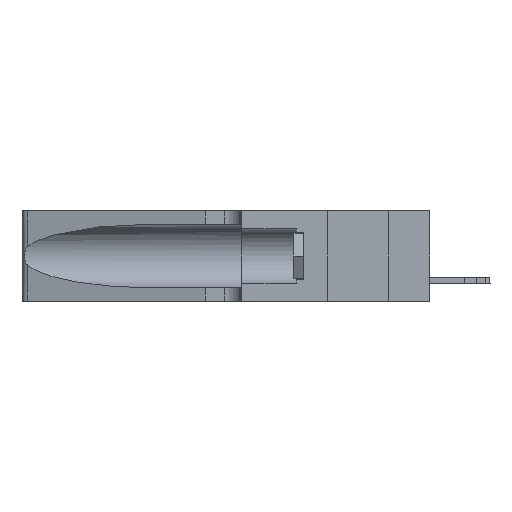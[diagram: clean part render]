
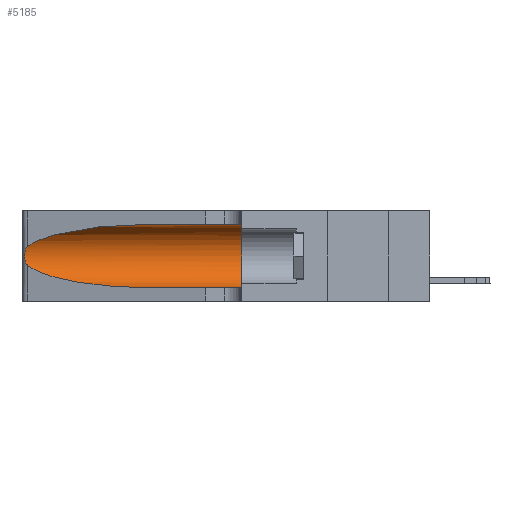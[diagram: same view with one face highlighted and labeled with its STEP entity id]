
A CAD part, left-side view. The second image highlights one B-rep face of the part: STEP entity #5185.
In plain terms, the highlighted cylindrical face has radius 3.308 mm (diameter 6.617 mm), a partial arc.
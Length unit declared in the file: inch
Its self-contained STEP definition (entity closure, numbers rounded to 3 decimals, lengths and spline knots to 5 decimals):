
#22 = CARTESIAN_POINT ( 'NONE',  ( 0.25789, 1.23486, 0.15765 ) ) ;
#763 = DIRECTION ( 'NONE',  ( 0., -1., 0. ) ) ;
#1405 = ORIENTED_EDGE ( 'NONE', *, *, #16992, .T. ) ;
#1784 = CYLINDRICAL_SURFACE ( 'NONE', #16320, 0.13025 ) ;
#2028 = CARTESIAN_POINT ( 'NONE',  ( 0.1305, 0.72297, 0.31525 ) ) ;
#2311 = VECTOR ( 'NONE', #4547, 39.37008 ) ;
#2372 = CARTESIAN_POINT ( 'NONE',  ( 0.25487, 1.22718, 0.22369 ) ) ;
#2548 = EDGE_CURVE ( 'NONE', #8157, #13876, #9603, .T. ) ;
#2886 = CARTESIAN_POINT ( 'NONE',  ( 0.2373, 1.15595, 0.08982 ) ) ;
#3053 = CARTESIAN_POINT ( 'NONE',  ( 0.1305, 0.72297, 0.05475 ) ) ;
#3152 = CARTESIAN_POINT ( 'NONE',  ( 0.18966, 0.96281, 0.05475 ) ) ;
#3193 = EDGE_CURVE ( 'NONE', #5038, #15897, #12109, .T. ) ;
#4183 = EDGE_CURVE ( 'NONE', #26659, #13906, #15864, .T. ) ;
#4516 = CARTESIAN_POINT ( 'NONE',  ( 0.25555, 1.22994, 0.2215 ) ) ;
#4547 = DIRECTION ( 'NONE',  ( 0., -1., 0. ) ) ;
#5038 = VERTEX_POINT ( 'NONE', #2028 ) ;
#5119 = B_SPLINE_CURVE_WITH_KNOTS ( 'NONE', 3,
 ( #2372, #4516, #8819, #21678, #25869, #15315, #19639, #6875, #10664, #25597, #22, #13448, #9180, #19827 ),
 .UNSPECIFIED., .F., .F.,
 ( 4, 2, 2, 2, 2, 2, 4 ),
 ( 0., 0.00027, 0.00053, 0.00107, 0.0016, 0.00187, 0.00214 ),
 .UNSPECIFIED. ) ;
#5185 = ADVANCED_FACE ( 'NONE', ( #24451 ), #1784, .F. ) ;
#5332 = CARTESIAN_POINT ( 'NONE',  ( 0.1305, 0.35, 0.185 ) ) ;
#6429 = CARTESIAN_POINT ( 'NONE',  ( 0.1305, 1.61858, 0.185 ) ) ;
#6658 = EDGE_CURVE ( 'NONE', #13906, #13876, #23361, .T. ) ;
#6875 = CARTESIAN_POINT ( 'NONE',  ( 0.26075, 1.23896, 0.178 ) ) ;
#7969 = ORIENTED_EDGE ( 'NONE', *, *, #6658, .T. ) ;
#8107 = ORIENTED_EDGE ( 'NONE', *, *, #2548, .F. ) ;
#8157 = VERTEX_POINT ( 'NONE', #8378 ) ;
#8378 = CARTESIAN_POINT ( 'NONE',  ( 0.1305, 0.35, 0.31525 ) ) ;
#8819 = CARTESIAN_POINT ( 'NONE',  ( 0.25639, 1.23184, 0.21858 ) ) ;
#9180 = CARTESIAN_POINT ( 'NONE',  ( 0.25555, 1.22993, 0.14849 ) ) ;
#9235 = CARTESIAN_POINT ( 'NONE',  ( 0.1305, 0.72297, 0.05475 ) ) ;
#9506 = CARTESIAN_POINT ( 'NONE',  ( 0.1305, 0.35, 0.05475 ) ) ;
#9532 = AXIS2_PLACEMENT_3D ( 'NONE', #5332, #13812, #20190 ) ;
#9603 = CIRCLE ( 'NONE', #9532, 0.13025 ) ;
#10664 = CARTESIAN_POINT ( 'NONE',  ( 0.26017, 1.23833, 0.17102 ) ) ;
#10693 = CARTESIAN_POINT ( 'NONE',  ( 0.25487, 1.22718, 0.22369 ) ) ;
#10745 = CARTESIAN_POINT ( 'NONE',  ( 0.1305, 1.61858, 0.05475 ) ) ;
#10789 = CARTESIAN_POINT ( 'NONE',  ( 0.1305, 1.61858, 0.31525 ) ) ;
#12109 =( BOUNDED_CURVE ( )  B_SPLINE_CURVE ( 3, ( #15170, #23461, #21613, #10693 ),
 .UNSPECIFIED., .F., .F. ) 
 B_SPLINE_CURVE_WITH_KNOTS ( ( 4, 4 ),
 ( 1.5708, 2.84003 ),
 .UNSPECIFIED. ) 
 CURVE ( )  GEOMETRIC_REPRESENTATION_ITEM ( )  RATIONAL_B_SPLINE_CURVE ( ( 1., 0.87, 0.87, 1. ) ) 
 REPRESENTATION_ITEM ( '' )  );
#12924 = DIRECTION ( 'NONE',  ( 0., 0., -1. ) ) ;
#13448 = CARTESIAN_POINT ( 'NONE',  ( 0.25639, 1.23186, 0.15144 ) ) ;
#13812 = DIRECTION ( 'NONE',  ( 0., 1., 0. ) ) ;
#13876 = VERTEX_POINT ( 'NONE', #9506 ) ;
#13906 = VERTEX_POINT ( 'NONE', #3053 ) ;
#14595 = CARTESIAN_POINT ( 'NONE',  ( 0.25487, 1.22718, 0.22369 ) ) ;
#15170 = CARTESIAN_POINT ( 'NONE',  ( 0.1305, 0.72297, 0.31525 ) ) ;
#15315 = CARTESIAN_POINT ( 'NONE',  ( 0.26018, 1.23835, 0.19895 ) ) ;
#15864 =( BOUNDED_CURVE ( )  B_SPLINE_CURVE ( 3, ( #22086, #2886, #3152, #9235 ),
 .UNSPECIFIED., .F., .F. ) 
 B_SPLINE_CURVE_WITH_KNOTS ( ( 4, 4 ),
 ( 3.44316, 4.71239 ),
 .UNSPECIFIED. ) 
 CURVE ( )  GEOMETRIC_REPRESENTATION_ITEM ( )  RATIONAL_B_SPLINE_CURVE ( ( 1., 0.87, 0.87, 1. ) ) 
 REPRESENTATION_ITEM ( '' )  );
#15897 = VERTEX_POINT ( 'NONE', #14595 ) ;
#16119 = EDGE_CURVE ( 'NONE', #5038, #8157, #26332, .T. ) ;
#16320 = AXIS2_PLACEMENT_3D ( 'NONE', #6429, #17195, #12924 ) ;
#16992 = EDGE_CURVE ( 'NONE', #15897, #26659, #5119, .T. ) ;
#17195 = DIRECTION ( 'NONE',  ( 0., -1., 0. ) ) ;
#18095 = CARTESIAN_POINT ( 'NONE',  ( 0.25487, 1.22718, 0.14631 ) ) ;
#19639 = CARTESIAN_POINT ( 'NONE',  ( 0.26075, 1.23896, 0.19203 ) ) ;
#19740 = VECTOR ( 'NONE', #763, 39.37008 ) ;
#19827 = CARTESIAN_POINT ( 'NONE',  ( 0.25487, 1.22718, 0.14631 ) ) ;
#19957 = ORIENTED_EDGE ( 'NONE', *, *, #16119, .F. ) ;
#20163 = ORIENTED_EDGE ( 'NONE', *, *, #4183, .T. ) ;
#20190 = DIRECTION ( 'NONE',  ( 0., 0., 1. ) ) ;
#21613 = CARTESIAN_POINT ( 'NONE',  ( 0.2373, 1.15595, 0.28018 ) ) ;
#21678 = CARTESIAN_POINT ( 'NONE',  ( 0.25787, 1.23484, 0.2124 ) ) ;
#22086 = CARTESIAN_POINT ( 'NONE',  ( 0.25487, 1.22718, 0.14631 ) ) ;
#22320 = ORIENTED_EDGE ( 'NONE', *, *, #3193, .T. ) ;
#22358 = EDGE_LOOP ( 'NONE', ( #22320, #1405, #20163, #7969, #8107, #19957 ) ) ;
#23361 = LINE ( 'NONE', #10745, #19740 ) ;
#23461 = CARTESIAN_POINT ( 'NONE',  ( 0.18966, 0.96281, 0.31525 ) ) ;
#24451 = FACE_OUTER_BOUND ( 'NONE', #22358, .T. ) ;
#25597 = CARTESIAN_POINT ( 'NONE',  ( 0.25856, 1.23593, 0.16098 ) ) ;
#25869 = CARTESIAN_POINT ( 'NONE',  ( 0.25854, 1.2359, 0.20912 ) ) ;
#26332 = LINE ( 'NONE', #10789, #2311 ) ;
#26659 = VERTEX_POINT ( 'NONE', #18095 ) ;
